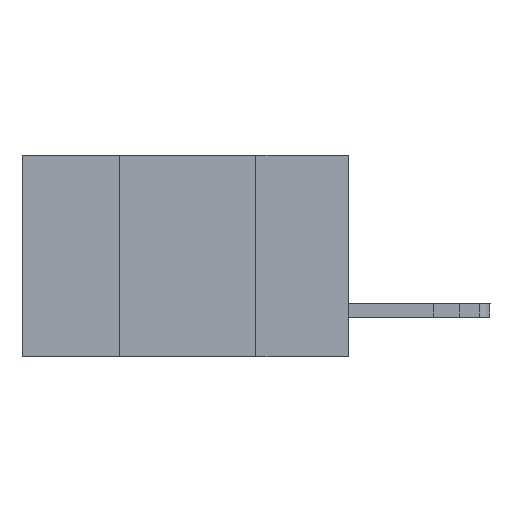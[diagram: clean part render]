
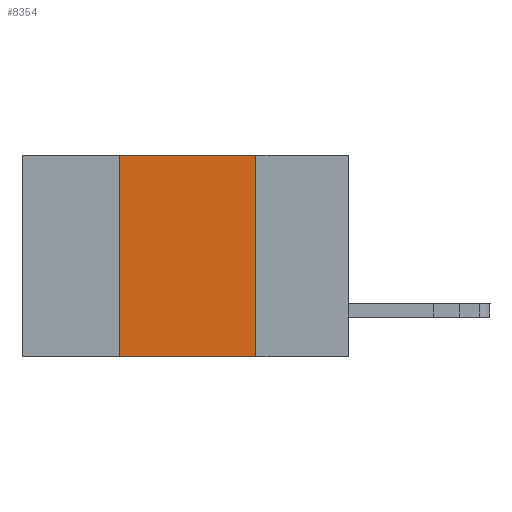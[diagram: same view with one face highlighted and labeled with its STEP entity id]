
A CAD part, left-side view. The second image highlights one B-rep face of the part: STEP entity #8354.
In plain terms, the highlighted planar face has unit normal (-1, 0, 0).
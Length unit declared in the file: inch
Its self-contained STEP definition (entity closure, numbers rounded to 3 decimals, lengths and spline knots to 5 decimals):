
#369 = ORIENTED_EDGE ( 'NONE', *, *, #18020, .F. ) ;
#1096 = EDGE_CURVE ( 'NONE', #6480, #4344, #13597, .T. ) ;
#2123 = DIRECTION ( 'NONE',  ( 0., -1., 0. ) ) ;
#3507 = FACE_OUTER_BOUND ( 'NONE', #11692, .T. ) ;
#4344 = VERTEX_POINT ( 'NONE', #12162 ) ;
#4775 = CARTESIAN_POINT ( 'NONE',  ( 0., 0.6, 0. ) ) ;
#4893 = VECTOR ( 'NONE', #8726, 39.37008 ) ;
#5576 = CARTESIAN_POINT ( 'NONE',  ( 0., 0.42, -0.37 ) ) ;
#6342 = CARTESIAN_POINT ( 'NONE',  ( 0., 0.42, -0.37 ) ) ;
#6480 = VERTEX_POINT ( 'NONE', #12341 ) ;
#6490 = DIRECTION ( 'NONE',  ( 0., -1., 0. ) ) ;
#7200 = CARTESIAN_POINT ( 'NONE',  ( 0., 0.42, 0. ) ) ;
#7222 = LINE ( 'NONE', #5576, #11579 ) ;
#7711 = LINE ( 'NONE', #13751, #19899 ) ;
#7858 = VERTEX_POINT ( 'NONE', #7200 ) ;
#8054 = ORIENTED_EDGE ( 'NONE', *, *, #21127, .F. ) ;
#8354 = ADVANCED_FACE ( 'NONE', ( #3507 ), #11013, .F. ) ;
#8726 = DIRECTION ( 'NONE',  ( 0., 0., -1. ) ) ;
#8844 = CARTESIAN_POINT ( 'NONE',  ( 0., 0.17, -0.37 ) ) ;
#10750 = VECTOR ( 'NONE', #6490, 39.37008 ) ;
#10842 = DIRECTION ( 'NONE',  ( 0., 0., -1. ) ) ;
#10886 = DIRECTION ( 'NONE',  ( 1., 0., 0. ) ) ;
#10929 = CARTESIAN_POINT ( 'NONE',  ( 0., 0.6, 0. ) ) ;
#11013 = PLANE ( 'NONE',  #16354 ) ;
#11579 = VECTOR ( 'NONE', #16856, 39.37008 ) ;
#11692 = EDGE_LOOP ( 'NONE', ( #14211, #8054, #369, #18524 ) ) ;
#12162 = CARTESIAN_POINT ( 'NONE',  ( 0., 0.17, -0.37 ) ) ;
#12341 = CARTESIAN_POINT ( 'NONE',  ( 0., 0.17, 0. ) ) ;
#13597 = LINE ( 'NONE', #8844, #4893 ) ;
#13751 = CARTESIAN_POINT ( 'NONE',  ( 0., 0.6, -0.37 ) ) ;
#14211 = ORIENTED_EDGE ( 'NONE', *, *, #1096, .F. ) ;
#16354 = AXIS2_PLACEMENT_3D ( 'NONE', #10929, #10886, #10842 ) ;
#16856 = DIRECTION ( 'NONE',  ( 0., 0., 1. ) ) ;
#18020 = EDGE_CURVE ( 'NONE', #19059, #7858, #7222, .T. ) ;
#18524 = ORIENTED_EDGE ( 'NONE', *, *, #20500, .T. ) ;
#19059 = VERTEX_POINT ( 'NONE', #6342 ) ;
#19148 = LINE ( 'NONE', #4775, #10750 ) ;
#19899 = VECTOR ( 'NONE', #2123, 39.37008 ) ;
#20500 = EDGE_CURVE ( 'NONE', #19059, #4344, #7711, .T. ) ;
#21127 = EDGE_CURVE ( 'NONE', #7858, #6480, #19148, .T. ) ;
